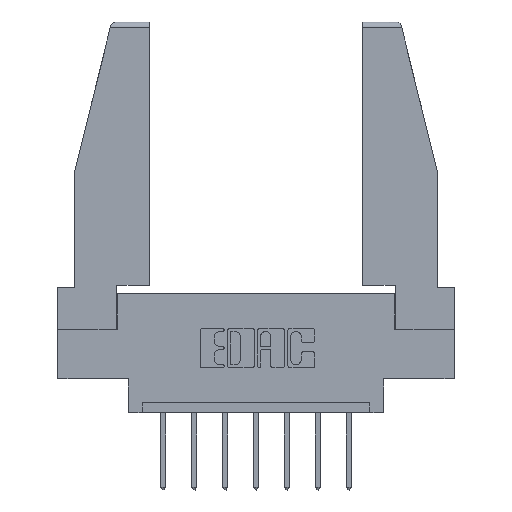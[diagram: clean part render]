
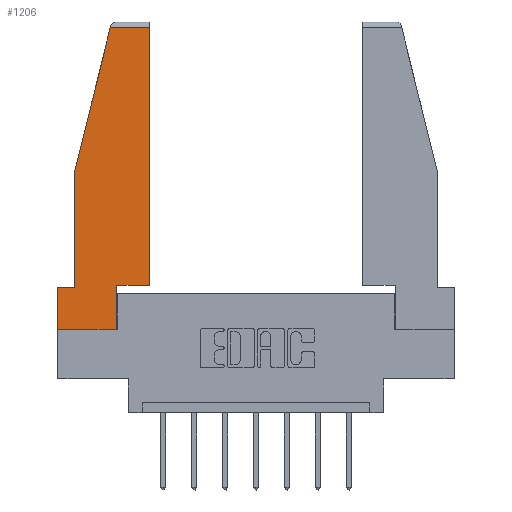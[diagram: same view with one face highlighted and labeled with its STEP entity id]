
A CAD part, top view. The second image highlights one B-rep face of the part: STEP entity #1206.
In plain terms, the highlighted planar face has unit normal (0, 0, 1).
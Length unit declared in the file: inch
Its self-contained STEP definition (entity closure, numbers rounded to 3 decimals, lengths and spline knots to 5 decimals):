
#6 = CARTESIAN_POINT ( 'NONE',  ( 0.271, 1.55, 0. ) ) ;
#147 = VECTOR ( 'NONE', #9484, 39.37008 ) ;
#150 = ORIENTED_EDGE ( 'NONE', *, *, #9835, .T. ) ;
#495 = VERTEX_POINT ( 'NONE', #11516 ) ;
#876 = DIRECTION ( 'NONE',  ( 0., 1., 0. ) ) ;
#1001 = VERTEX_POINT ( 'NONE', #11630 ) ;
#1070 = CARTESIAN_POINT ( 'NONE',  ( 0.297, 0.223, 0. ) ) ;
#1102 = CARTESIAN_POINT ( 'NONE',  ( 0., 1.52, 0. ) ) ;
#1138 = EDGE_LOOP ( 'NONE', ( #4268, #1702, #7482, #11296, #3956, #5133, #3367, #11114, #150 ) ) ;
#1206 = ADVANCED_FACE ( 'NONE', ( #9392 ), #12342, .T. ) ;
#1350 = DIRECTION ( 'NONE',  ( 1., 0., 0. ) ) ;
#1408 = CARTESIAN_POINT ( 'NONE',  ( 0.2636, 1.52, 0. ) ) ;
#1431 = LINE ( 'NONE', #4669, #1883 ) ;
#1577 = VERTEX_POINT ( 'NONE', #9064 ) ;
#1702 = ORIENTED_EDGE ( 'NONE', *, *, #1730, .T. ) ;
#1730 = EDGE_CURVE ( 'NONE', #7866, #9271, #9831, .T. ) ;
#1883 = VECTOR ( 'NONE', #2714, 39.37008 ) ;
#1890 = DIRECTION ( 'NONE',  ( 0., 0., 1. ) ) ;
#2618 = CARTESIAN_POINT ( 'NONE',  ( 0., 0.21, 0. ) ) ;
#2714 = DIRECTION ( 'NONE',  ( 0., 1., 0. ) ) ;
#3041 = CARTESIAN_POINT ( 'NONE',  ( 0.461, 1.52, 0. ) ) ;
#3088 = CARTESIAN_POINT ( 'NONE',  ( 0.086, 0.8, 0. ) ) ;
#3367 = ORIENTED_EDGE ( 'NONE', *, *, #5033, .T. ) ;
#3387 = LINE ( 'NONE', #1070, #3683 ) ;
#3479 = CARTESIAN_POINT ( 'NONE',  ( 0., 0.21, 0. ) ) ;
#3683 = VECTOR ( 'NONE', #1350, 39.37008 ) ;
#3718 = VERTEX_POINT ( 'NONE', #10720 ) ;
#3956 = ORIENTED_EDGE ( 'NONE', *, *, #8208, .T. ) ;
#4268 = ORIENTED_EDGE ( 'NONE', *, *, #8372, .T. ) ;
#4639 = LINE ( 'NONE', #3479, #5672 ) ;
#4669 = CARTESIAN_POINT ( 'NONE',  ( 0.297, 0., 0. ) ) ;
#4691 = CARTESIAN_POINT ( 'NONE',  ( 0.461, 0.223, 0. ) ) ;
#4820 = DIRECTION ( 'NONE',  ( -1., 0., 0. ) ) ;
#5033 = EDGE_CURVE ( 'NONE', #495, #7541, #9465, .T. ) ;
#5133 = ORIENTED_EDGE ( 'NONE', *, *, #11498, .T. ) ;
#5491 = EDGE_CURVE ( 'NONE', #7541, #1001, #1431, .T. ) ;
#5554 = DIRECTION ( 'NONE',  ( -1., 0., 0. ) ) ;
#5672 = VECTOR ( 'NONE', #5554, 39.37008 ) ;
#6391 = LINE ( 'NONE', #8491, #147 ) ;
#6547 = VECTOR ( 'NONE', #12042, 39.37008 ) ;
#6605 = CARTESIAN_POINT ( 'NONE',  ( 0., 0., 0. ) ) ;
#7140 = LINE ( 'NONE', #6, #9232 ) ;
#7482 = ORIENTED_EDGE ( 'NONE', *, *, #8892, .T. ) ;
#7541 = VERTEX_POINT ( 'NONE', #8234 ) ;
#7866 = VERTEX_POINT ( 'NONE', #3041 ) ;
#8208 = EDGE_CURVE ( 'NONE', #1577, #3718, #4639, .T. ) ;
#8234 = CARTESIAN_POINT ( 'NONE',  ( 0.297, 0., 0. ) ) ;
#8372 = EDGE_CURVE ( 'NONE', #11637, #7866, #10148, .T. ) ;
#8413 = CARTESIAN_POINT ( 'NONE',  ( 0.461, 0.223, 0. ) ) ;
#8491 = CARTESIAN_POINT ( 'NONE',  ( 0.086, 0.8, 0. ) ) ;
#8529 = DIRECTION ( 'NONE',  ( 1., 0., 0. ) ) ;
#8610 = DIRECTION ( 'NONE',  ( -0.239, -0.971, 0. ) ) ;
#8628 = AXIS2_PLACEMENT_3D ( 'NONE', #6605, #1890, #8529 ) ;
#8892 = EDGE_CURVE ( 'NONE', #9271, #10979, #7140, .T. ) ;
#9064 = CARTESIAN_POINT ( 'NONE',  ( 0.086, 0.21, 0. ) ) ;
#9072 = LINE ( 'NONE', #2618, #6547 ) ;
#9148 = EDGE_CURVE ( 'NONE', #10979, #1577, #6391, .T. ) ;
#9232 = VECTOR ( 'NONE', #8610, 39.37008 ) ;
#9271 = VERTEX_POINT ( 'NONE', #1408 ) ;
#9293 = DIRECTION ( 'NONE',  ( 1., 0., 0. ) ) ;
#9392 = FACE_OUTER_BOUND ( 'NONE', #1138, .T. ) ;
#9465 = LINE ( 'NONE', #12232, #10691 ) ;
#9484 = DIRECTION ( 'NONE',  ( 0., -1., 0. ) ) ;
#9831 = LINE ( 'NONE', #1102, #11338 ) ;
#9835 = EDGE_CURVE ( 'NONE', #1001, #11637, #3387, .T. ) ;
#10148 = LINE ( 'NONE', #4691, #11352 ) ;
#10691 = VECTOR ( 'NONE', #9293, 39.37008 ) ;
#10720 = CARTESIAN_POINT ( 'NONE',  ( 0., 0.21, 0. ) ) ;
#10979 = VERTEX_POINT ( 'NONE', #3088 ) ;
#11114 = ORIENTED_EDGE ( 'NONE', *, *, #5491, .T. ) ;
#11296 = ORIENTED_EDGE ( 'NONE', *, *, #9148, .T. ) ;
#11338 = VECTOR ( 'NONE', #4820, 39.37008 ) ;
#11352 = VECTOR ( 'NONE', #876, 39.37008 ) ;
#11498 = EDGE_CURVE ( 'NONE', #3718, #495, #9072, .T. ) ;
#11516 = CARTESIAN_POINT ( 'NONE',  ( 0., 0., 0. ) ) ;
#11630 = CARTESIAN_POINT ( 'NONE',  ( 0.297, 0.223, 0. ) ) ;
#11637 = VERTEX_POINT ( 'NONE', #8413 ) ;
#12042 = DIRECTION ( 'NONE',  ( 0., -1., 0. ) ) ;
#12232 = CARTESIAN_POINT ( 'NONE',  ( 0., 0., 0. ) ) ;
#12342 = PLANE ( 'NONE',  #8628 ) ;
